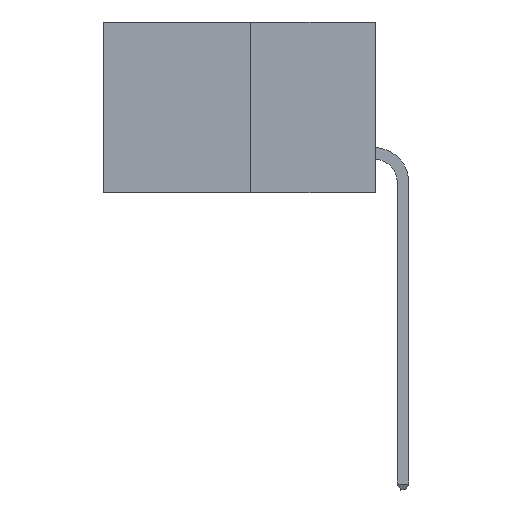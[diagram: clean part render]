
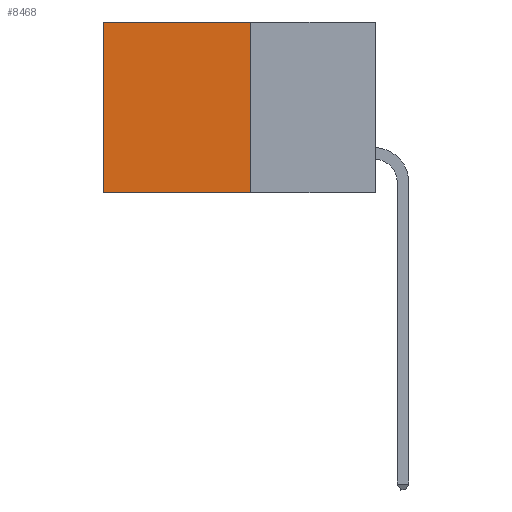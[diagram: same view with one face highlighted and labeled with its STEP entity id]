
A CAD part, left-side view. The second image highlights one B-rep face of the part: STEP entity #8468.
In plain terms, the highlighted planar face has unit normal (-1, 0, 0).
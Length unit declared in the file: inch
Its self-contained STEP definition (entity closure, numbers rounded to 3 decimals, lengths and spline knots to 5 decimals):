
#223 = CARTESIAN_POINT ( 'NONE',  ( 0.277, 0.27, 0. ) ) ;
#635 = ORIENTED_EDGE ( 'NONE', *, *, #1846, .T. ) ;
#822 = EDGE_LOOP ( 'NONE', ( #8592, #3463, #11407, #635 ) ) ;
#1443 = CARTESIAN_POINT ( 'NONE',  ( 0.277, 0.59, 0. ) ) ;
#1509 = CARTESIAN_POINT ( 'NONE',  ( 0.277, 0.27, -0.37 ) ) ;
#1800 = LINE ( 'NONE', #7013, #10024 ) ;
#1846 = EDGE_CURVE ( 'NONE', #9625, #10583, #8641, .T. ) ;
#1928 = DIRECTION ( 'NONE',  ( 0., 1., 0. ) ) ;
#2461 = DIRECTION ( 'NONE',  ( 1., 0., 0. ) ) ;
#2944 = VERTEX_POINT ( 'NONE', #8714 ) ;
#3463 = ORIENTED_EDGE ( 'NONE', *, *, #5212, .F. ) ;
#5212 = EDGE_CURVE ( 'NONE', #2944, #6759, #7310, .T. ) ;
#6635 = PLANE ( 'NONE',  #13086 ) ;
#6759 = VERTEX_POINT ( 'NONE', #9391 ) ;
#6870 = FACE_OUTER_BOUND ( 'NONE', #822, .T. ) ;
#7013 = CARTESIAN_POINT ( 'NONE',  ( 0.277, 0.59, -0.37 ) ) ;
#7310 = LINE ( 'NONE', #1509, #12411 ) ;
#8025 = VECTOR ( 'NONE', #11877, 39.37008 ) ;
#8468 = ADVANCED_FACE ( 'NONE', ( #6870 ), #6635, .F. ) ;
#8592 = ORIENTED_EDGE ( 'NONE', *, *, #12102, .T. ) ;
#8641 = LINE ( 'NONE', #11862, #8025 ) ;
#8647 = CARTESIAN_POINT ( 'NONE',  ( 0.277, 0.27, -0.37 ) ) ;
#8714 = CARTESIAN_POINT ( 'NONE',  ( 0.277, 0.27, -0.37 ) ) ;
#8982 = CARTESIAN_POINT ( 'NONE',  ( 0.277, 0.27, -0.37 ) ) ;
#9391 = CARTESIAN_POINT ( 'NONE',  ( 0.277, 0.59, -0.37 ) ) ;
#9571 = DIRECTION ( 'NONE',  ( 0., 0., -1. ) ) ;
#9625 = VERTEX_POINT ( 'NONE', #223 ) ;
#9696 = EDGE_CURVE ( 'NONE', #9625, #2944, #10831, .T. ) ;
#9922 = DIRECTION ( 'NONE',  ( 0., 0., -1. ) ) ;
#10024 = VECTOR ( 'NONE', #12749, 39.37008 ) ;
#10583 = VERTEX_POINT ( 'NONE', #1443 ) ;
#10831 = LINE ( 'NONE', #8982, #13074 ) ;
#11407 = ORIENTED_EDGE ( 'NONE', *, *, #9696, .F. ) ;
#11862 = CARTESIAN_POINT ( 'NONE',  ( 0.277, 0.27, 0. ) ) ;
#11877 = DIRECTION ( 'NONE',  ( 0., 1., 0. ) ) ;
#12102 = EDGE_CURVE ( 'NONE', #10583, #6759, #1800, .T. ) ;
#12411 = VECTOR ( 'NONE', #1928, 39.37008 ) ;
#12749 = DIRECTION ( 'NONE',  ( 0., 0., -1. ) ) ;
#13074 = VECTOR ( 'NONE', #9922, 39.37008 ) ;
#13086 = AXIS2_PLACEMENT_3D ( 'NONE', #8647, #2461, #9571 ) ;
